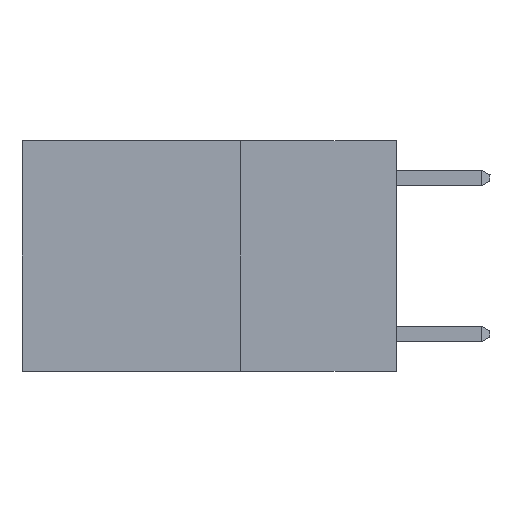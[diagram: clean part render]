
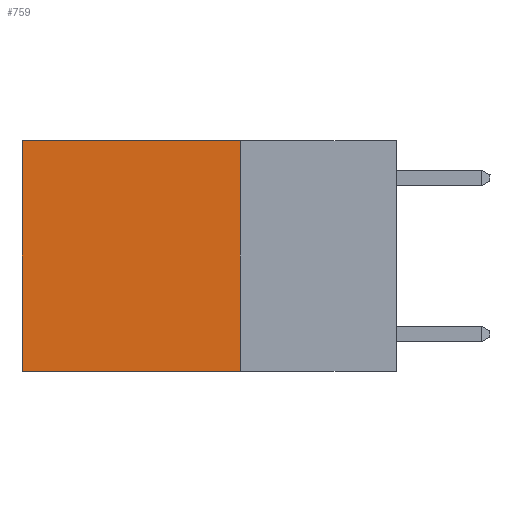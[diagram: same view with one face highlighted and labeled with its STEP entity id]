
A CAD part, left-side view. The second image highlights one B-rep face of the part: STEP entity #759.
In plain terms, the highlighted planar face has unit normal (-1, 0, 0).
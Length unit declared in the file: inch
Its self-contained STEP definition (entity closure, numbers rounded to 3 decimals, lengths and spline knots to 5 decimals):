
#13 = DIRECTION ( 'NONE',  ( 0., 1., 0. ) ) ;
#46 = VECTOR ( 'NONE', #13, 39.37008 ) ;
#120 = EDGE_LOOP ( 'NONE', ( #2829, #6484, #273, #2380 ) ) ;
#273 = ORIENTED_EDGE ( 'NONE', *, *, #1456, .F. ) ;
#644 = CARTESIAN_POINT ( 'NONE',  ( 0.2625, 0.25, 0. ) ) ;
#680 = DIRECTION ( 'NONE',  ( 0., 1., 0. ) ) ;
#759 = ADVANCED_FACE ( 'NONE', ( #6986 ), #3764, .F. ) ;
#949 = VERTEX_POINT ( 'NONE', #7357 ) ;
#1009 = DIRECTION ( 'NONE',  ( 0., 0., -1. ) ) ;
#1168 = CARTESIAN_POINT ( 'NONE',  ( 0.2625, 0.6, 0. ) ) ;
#1456 = EDGE_CURVE ( 'NONE', #949, #6679, #4845, .T. ) ;
#1842 = EDGE_CURVE ( 'NONE', #6679, #5903, #6487, .T. ) ;
#2028 = CARTESIAN_POINT ( 'NONE',  ( 0.2625, 0.25, -0.37 ) ) ;
#2220 = EDGE_CURVE ( 'NONE', #949, #7199, #6450, .T. ) ;
#2257 = CARTESIAN_POINT ( 'NONE',  ( 0.2625, 0.25, -0.37 ) ) ;
#2380 = ORIENTED_EDGE ( 'NONE', *, *, #2220, .T. ) ;
#2746 = DIRECTION ( 'NONE',  ( 0., 0., -1. ) ) ;
#2829 = ORIENTED_EDGE ( 'NONE', *, *, #7243, .T. ) ;
#3168 = VECTOR ( 'NONE', #2746, 39.37008 ) ;
#3764 = PLANE ( 'NONE',  #8286 ) ;
#3880 = CARTESIAN_POINT ( 'NONE',  ( 0.2625, 0.6, -0.37 ) ) ;
#4343 = DIRECTION ( 'NONE',  ( 1., 0., 0. ) ) ;
#4845 = LINE ( 'NONE', #6727, #4921 ) ;
#4921 = VECTOR ( 'NONE', #1009, 39.37008 ) ;
#5197 = VECTOR ( 'NONE', #680, 39.37008 ) ;
#5198 = LINE ( 'NONE', #6466, #3168 ) ;
#5903 = VERTEX_POINT ( 'NONE', #3880 ) ;
#6336 = DIRECTION ( 'NONE',  ( 0., 0., -1. ) ) ;
#6369 = CARTESIAN_POINT ( 'NONE',  ( 0.2625, 0.25, 0. ) ) ;
#6450 = LINE ( 'NONE', #644, #46 ) ;
#6466 = CARTESIAN_POINT ( 'NONE',  ( 0.2625, 0.6, 0. ) ) ;
#6484 = ORIENTED_EDGE ( 'NONE', *, *, #1842, .F. ) ;
#6487 = LINE ( 'NONE', #2028, #5197 ) ;
#6679 = VERTEX_POINT ( 'NONE', #2257 ) ;
#6727 = CARTESIAN_POINT ( 'NONE',  ( 0.2625, 0.25, 0. ) ) ;
#6986 = FACE_OUTER_BOUND ( 'NONE', #120, .T. ) ;
#7199 = VERTEX_POINT ( 'NONE', #1168 ) ;
#7243 = EDGE_CURVE ( 'NONE', #7199, #5903, #5198, .T. ) ;
#7357 = CARTESIAN_POINT ( 'NONE',  ( 0.2625, 0.25, 0. ) ) ;
#8286 = AXIS2_PLACEMENT_3D ( 'NONE', #6369, #4343, #6336 ) ;
